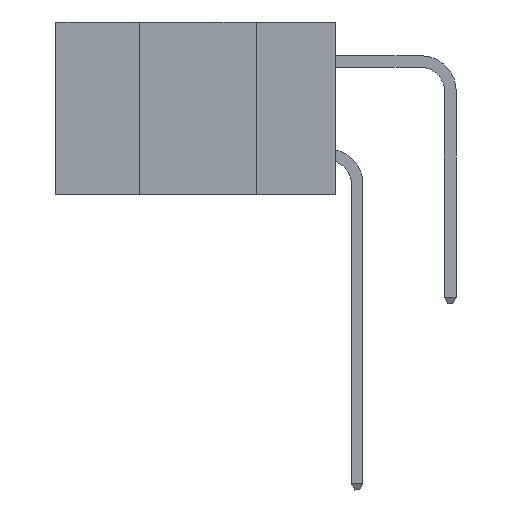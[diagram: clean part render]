
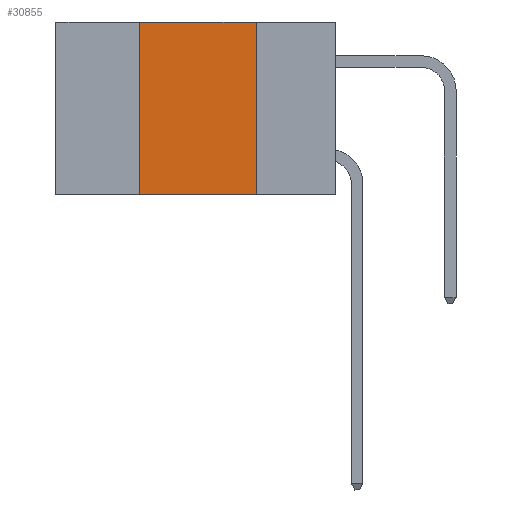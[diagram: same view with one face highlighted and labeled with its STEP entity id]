
A CAD part, left-side view. The second image highlights one B-rep face of the part: STEP entity #30855.
In plain terms, the highlighted planar face has unit normal (-1, 0, 0).
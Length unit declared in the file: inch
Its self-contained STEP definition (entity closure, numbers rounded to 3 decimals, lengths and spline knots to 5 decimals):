
#104 = EDGE_CURVE ( 'NONE', #25117, #5192, #31303, .T. ) ;
#653 = VERTEX_POINT ( 'NONE', #24758 ) ;
#755 = CARTESIAN_POINT ( 'NONE',  ( 0., 0.6, 0. ) ) ;
#962 = ORIENTED_EDGE ( 'NONE', *, *, #4861, .T. ) ;
#3089 = ORIENTED_EDGE ( 'NONE', *, *, #14738, .F. ) ;
#4861 = EDGE_CURVE ( 'NONE', #653, #31074, #13248, .T. ) ;
#4938 = EDGE_LOOP ( 'NONE', ( #3089, #6333, #15034, #962 ) ) ;
#5192 = VERTEX_POINT ( 'NONE', #22277 ) ;
#6333 = ORIENTED_EDGE ( 'NONE', *, *, #104, .F. ) ;
#6758 = FACE_OUTER_BOUND ( 'NONE', #4938, .T. ) ;
#7614 = AXIS2_PLACEMENT_3D ( 'NONE', #31680, #17406, #20187 ) ;
#8208 = CARTESIAN_POINT ( 'NONE',  ( 0., 0.42, 0. ) ) ;
#12899 = EDGE_CURVE ( 'NONE', #653, #25117, #23764, .T. ) ;
#13248 = LINE ( 'NONE', #15912, #25385 ) ;
#14077 = LINE ( 'NONE', #32850, #15815 ) ;
#14738 = EDGE_CURVE ( 'NONE', #5192, #31074, #14077, .T. ) ;
#15034 = ORIENTED_EDGE ( 'NONE', *, *, #12899, .F. ) ;
#15815 = VECTOR ( 'NONE', #22510, 39.37008 ) ;
#15912 = CARTESIAN_POINT ( 'NONE',  ( 0., 0.6, -0.37 ) ) ;
#17406 = DIRECTION ( 'NONE',  ( 1., 0., 0. ) ) ;
#20187 = DIRECTION ( 'NONE',  ( 0., 0., -1. ) ) ;
#20411 = DIRECTION ( 'NONE',  ( 0., -1., 0. ) ) ;
#22277 = CARTESIAN_POINT ( 'NONE',  ( 0., 0.17, 0. ) ) ;
#22510 = DIRECTION ( 'NONE',  ( 0., 0., -1. ) ) ;
#23764 = LINE ( 'NONE', #8208, #32883 ) ;
#24758 = CARTESIAN_POINT ( 'NONE',  ( 0., 0.42, -0.37 ) ) ;
#25117 = VERTEX_POINT ( 'NONE', #29598 ) ;
#25385 = VECTOR ( 'NONE', #29610, 39.37008 ) ;
#27498 = CARTESIAN_POINT ( 'NONE',  ( 0., 0.17, -0.37 ) ) ;
#29598 = CARTESIAN_POINT ( 'NONE',  ( 0., 0.42, 0. ) ) ;
#29610 = DIRECTION ( 'NONE',  ( 0., -1., 0. ) ) ;
#30855 = ADVANCED_FACE ( 'NONE', ( #6758 ), #31445, .F. ) ;
#31074 = VERTEX_POINT ( 'NONE', #27498 ) ;
#31303 = LINE ( 'NONE', #755, #32151 ) ;
#31445 = PLANE ( 'NONE',  #7614 ) ;
#31680 = CARTESIAN_POINT ( 'NONE',  ( 0., 0.6, 0. ) ) ;
#32151 = VECTOR ( 'NONE', #20411, 39.37008 ) ;
#32850 = CARTESIAN_POINT ( 'NONE',  ( 0., 0.17, 0. ) ) ;
#32883 = VECTOR ( 'NONE', #33190, 39.37008 ) ;
#33190 = DIRECTION ( 'NONE',  ( 0., 0., 1. ) ) ;
